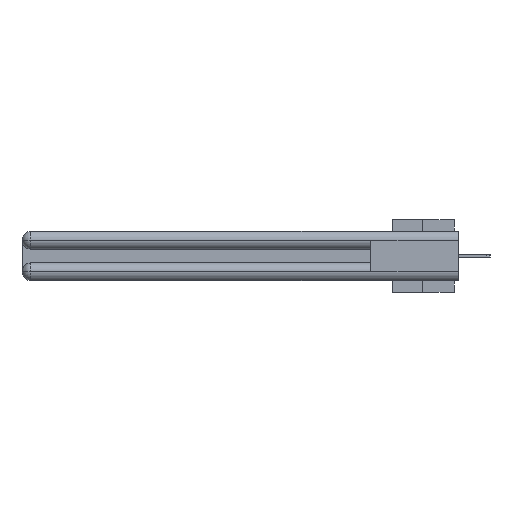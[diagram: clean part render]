
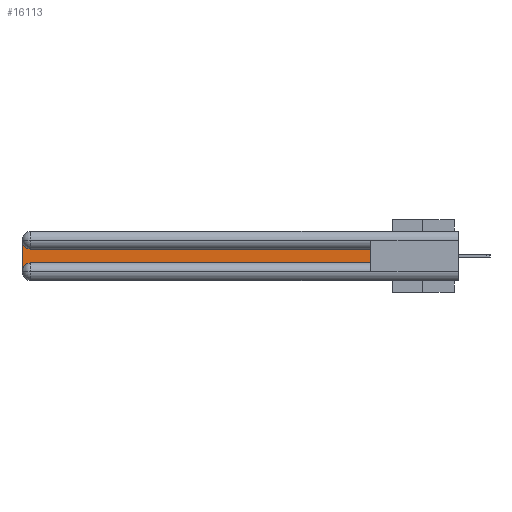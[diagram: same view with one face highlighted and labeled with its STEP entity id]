
A CAD part, left-side view. The second image highlights one B-rep face of the part: STEP entity #16113.
In plain terms, the highlighted planar face has unit normal (-1, 0, 0).
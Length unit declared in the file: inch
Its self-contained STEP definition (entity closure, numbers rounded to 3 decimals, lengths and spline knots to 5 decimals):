
#552 = CARTESIAN_POINT ( 'NONE',  ( 0.075, 3., -0.2775 ) ) ;
#1004 = EDGE_CURVE ( 'NONE', #10555, #26833, #22422, .T. ) ;
#1474 = CARTESIAN_POINT ( 'NONE',  ( 0.075, 0.6, -0.1225 ) ) ;
#2650 = ORIENTED_EDGE ( 'NONE', *, *, #15041, .T. ) ;
#2928 = EDGE_CURVE ( 'NONE', #10441, #9698, #13356, .T. ) ;
#4657 = LINE ( 'NONE', #32042, #18304 ) ;
#5326 = LINE ( 'NONE', #11509, #19796 ) ;
#5498 = DIRECTION ( 'NONE',  ( 1., 0., 0. ) ) ;
#5548 = CARTESIAN_POINT ( 'NONE',  ( 0.075, 2.94, -0.1225 ) ) ;
#8551 = VECTOR ( 'NONE', #22674, 39.37008 ) ;
#9466 = VERTEX_POINT ( 'NONE', #1474 ) ;
#9698 = VERTEX_POINT ( 'NONE', #10698 ) ;
#10441 = VERTEX_POINT ( 'NONE', #5548 ) ;
#10490 = VERTEX_POINT ( 'NONE', #27526 ) ;
#10555 = VERTEX_POINT ( 'NONE', #552 ) ;
#10698 = CARTESIAN_POINT ( 'NONE',  ( 0.075, 3., -0.0625 ) ) ;
#11509 = CARTESIAN_POINT ( 'NONE',  ( 0.075, 0.6, -0.1225 ) ) ;
#11583 = CARTESIAN_POINT ( 'NONE',  ( 0.075, 0.6, -0.2175 ) ) ;
#11851 = CARTESIAN_POINT ( 'NONE',  ( 0.075, 0.6, -0.2175 ) ) ;
#13355 = CARTESIAN_POINT ( 'NONE',  ( 0.075, 3., -0.1225 ) ) ;
#13356 = CIRCLE ( 'NONE', #32548, 0.06 ) ;
#14004 = AXIS2_PLACEMENT_3D ( 'NONE', #13355, #32360, #16134 ) ;
#14384 = DIRECTION ( 'NONE',  ( 0., 0., 1. ) ) ;
#15041 = EDGE_CURVE ( 'NONE', #9466, #10441, #5326, .T. ) ;
#16113 = ADVANCED_FACE ( 'NONE', ( #21845 ), #26890, .F. ) ;
#16134 = DIRECTION ( 'NONE',  ( 0., 0., -1. ) ) ;
#16668 = LINE ( 'NONE', #11851, #8551 ) ;
#17552 = EDGE_CURVE ( 'NONE', #26833, #10490, #16668, .T. ) ;
#18304 = VECTOR ( 'NONE', #34772, 39.37008 ) ;
#18571 = EDGE_LOOP ( 'NONE', ( #2650, #21594, #21936, #31134, #21215, #28090 ) ) ;
#19796 = VECTOR ( 'NONE', #25101, 39.37008 ) ;
#21215 = ORIENTED_EDGE ( 'NONE', *, *, #17552, .T. ) ;
#21594 = ORIENTED_EDGE ( 'NONE', *, *, #2928, .T. ) ;
#21795 = CARTESIAN_POINT ( 'NONE',  ( 0.075, 2.94, -0.0625 ) ) ;
#21845 = FACE_OUTER_BOUND ( 'NONE', #18571, .T. ) ;
#21936 = ORIENTED_EDGE ( 'NONE', *, *, #33713, .T. ) ;
#22422 = CIRCLE ( 'NONE', #25687, 0.06 ) ;
#22674 = DIRECTION ( 'NONE',  ( 0., -1., 0. ) ) ;
#24541 = DIRECTION ( 'NONE',  ( 0., 0., -1. ) ) ;
#25101 = DIRECTION ( 'NONE',  ( 0., 1., 0. ) ) ;
#25687 = AXIS2_PLACEMENT_3D ( 'NONE', #33413, #33363, #33570 ) ;
#26833 = VERTEX_POINT ( 'NONE', #35184 ) ;
#26890 = PLANE ( 'NONE',  #14004 ) ;
#27526 = CARTESIAN_POINT ( 'NONE',  ( 0.075, 0.6, -0.2175 ) ) ;
#28090 = ORIENTED_EDGE ( 'NONE', *, *, #32086, .T. ) ;
#29463 = VECTOR ( 'NONE', #14384, 39.37008 ) ;
#30334 = LINE ( 'NONE', #11583, #29463 ) ;
#31134 = ORIENTED_EDGE ( 'NONE', *, *, #1004, .T. ) ;
#32042 = CARTESIAN_POINT ( 'NONE',  ( 0.075, 3., -0.2175 ) ) ;
#32086 = EDGE_CURVE ( 'NONE', #10490, #9466, #30334, .T. ) ;
#32360 = DIRECTION ( 'NONE',  ( 1., 0., 0. ) ) ;
#32548 = AXIS2_PLACEMENT_3D ( 'NONE', #21795, #5498, #24541 ) ;
#33363 = DIRECTION ( 'NONE',  ( 1., 0., 0. ) ) ;
#33413 = CARTESIAN_POINT ( 'NONE',  ( 0.075, 2.94, -0.2775 ) ) ;
#33570 = DIRECTION ( 'NONE',  ( 0., 0., -1. ) ) ;
#33713 = EDGE_CURVE ( 'NONE', #9698, #10555, #4657, .T. ) ;
#34772 = DIRECTION ( 'NONE',  ( 0., 0., -1. ) ) ;
#35184 = CARTESIAN_POINT ( 'NONE',  ( 0.075, 2.94, -0.2175 ) ) ;
